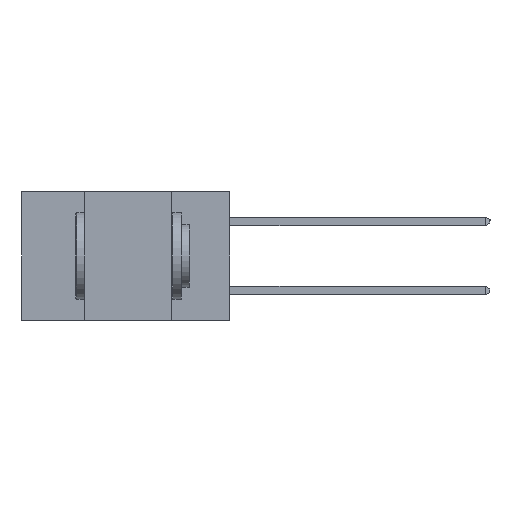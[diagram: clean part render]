
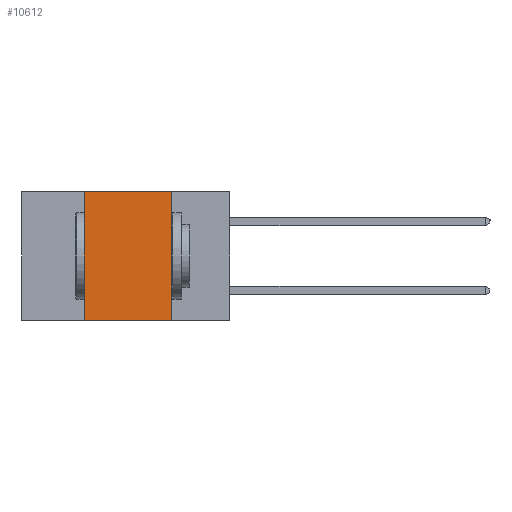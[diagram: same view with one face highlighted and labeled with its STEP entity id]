
A CAD part, left-side view. The second image highlights one B-rep face of the part: STEP entity #10612.
In plain terms, the highlighted planar face has unit normal (-1, 0, 0).
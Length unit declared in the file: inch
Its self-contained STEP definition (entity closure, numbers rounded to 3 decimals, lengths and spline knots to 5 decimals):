
#638 = AXIS2_PLACEMENT_3D ( 'NONE', #5321, #16407, #14190 ) ;
#3984 = CARTESIAN_POINT ( 'NONE',  ( 0., 0.6, -0.37 ) ) ;
#4045 = PLANE ( 'NONE',  #638 ) ;
#4497 = ORIENTED_EDGE ( 'NONE', *, *, #16665, .F. ) ;
#5321 = CARTESIAN_POINT ( 'NONE',  ( 0., 0.6, 0. ) ) ;
#6123 = LINE ( 'NONE', #6247, #17142 ) ;
#6247 = CARTESIAN_POINT ( 'NONE',  ( 0., 0.6, 0. ) ) ;
#6520 = CARTESIAN_POINT ( 'NONE',  ( 0., 0.17, -0.37 ) ) ;
#8282 = LINE ( 'NONE', #6520, #16228 ) ;
#8406 = VECTOR ( 'NONE', #11695, 39.37008 ) ;
#10612 = ADVANCED_FACE ( 'NONE', ( #21737 ), #4045, .F. ) ;
#11232 = CARTESIAN_POINT ( 'NONE',  ( 0., 0.17, -0.37 ) ) ;
#11695 = DIRECTION ( 'NONE',  ( 0., 0., 1. ) ) ;
#11784 = EDGE_CURVE ( 'NONE', #19069, #16444, #16460, .T. ) ;
#12144 = LINE ( 'NONE', #22847, #8406 ) ;
#12617 = EDGE_CURVE ( 'NONE', #13584, #19748, #6123, .T. ) ;
#13584 = VERTEX_POINT ( 'NONE', #22877 ) ;
#13842 = DIRECTION ( 'NONE',  ( 0., 0., -1. ) ) ;
#14190 = DIRECTION ( 'NONE',  ( 0., 0., -1. ) ) ;
#15102 = DIRECTION ( 'NONE',  ( 0., -1., 0. ) ) ;
#16228 = VECTOR ( 'NONE', #13842, 39.37008 ) ;
#16348 = ORIENTED_EDGE ( 'NONE', *, *, #17582, .F. ) ;
#16394 = EDGE_LOOP ( 'NONE', ( #16348, #19237, #4497, #21936 ) ) ;
#16407 = DIRECTION ( 'NONE',  ( 1., 0., 0. ) ) ;
#16444 = VERTEX_POINT ( 'NONE', #11232 ) ;
#16460 = LINE ( 'NONE', #3984, #22689 ) ;
#16665 = EDGE_CURVE ( 'NONE', #19069, #13584, #12144, .T. ) ;
#17142 = VECTOR ( 'NONE', #15102, 39.37008 ) ;
#17582 = EDGE_CURVE ( 'NONE', #19748, #16444, #8282, .T. ) ;
#17884 = CARTESIAN_POINT ( 'NONE',  ( 0., 0.42, -0.37 ) ) ;
#19069 = VERTEX_POINT ( 'NONE', #17884 ) ;
#19237 = ORIENTED_EDGE ( 'NONE', *, *, #12617, .F. ) ;
#19748 = VERTEX_POINT ( 'NONE', #20756 ) ;
#20071 = DIRECTION ( 'NONE',  ( 0., -1., 0. ) ) ;
#20756 = CARTESIAN_POINT ( 'NONE',  ( 0., 0.17, 0. ) ) ;
#21737 = FACE_OUTER_BOUND ( 'NONE', #16394, .T. ) ;
#21936 = ORIENTED_EDGE ( 'NONE', *, *, #11784, .T. ) ;
#22689 = VECTOR ( 'NONE', #20071, 39.37008 ) ;
#22847 = CARTESIAN_POINT ( 'NONE',  ( 0., 0.42, -0.37 ) ) ;
#22877 = CARTESIAN_POINT ( 'NONE',  ( 0., 0.42, 0. ) ) ;
